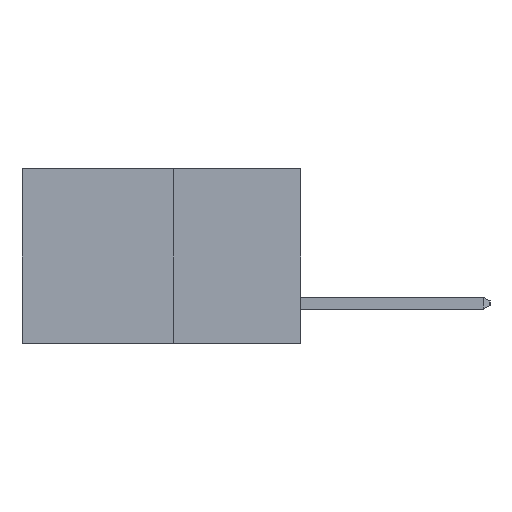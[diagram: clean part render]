
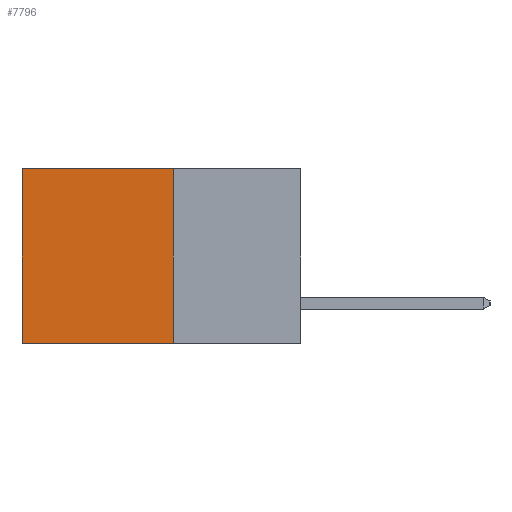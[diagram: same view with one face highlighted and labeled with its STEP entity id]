
A CAD part, left-side view. The second image highlights one B-rep face of the part: STEP entity #7796.
In plain terms, the highlighted planar face has unit normal (-1, 0, 0).
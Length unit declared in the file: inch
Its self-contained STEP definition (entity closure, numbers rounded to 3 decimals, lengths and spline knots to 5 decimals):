
#489 = LINE ( 'NONE', #5922, #3504 ) ;
#704 = LINE ( 'NONE', #11715, #1530 ) ;
#1110 = ORIENTED_EDGE ( 'NONE', *, *, #11844, .F. ) ;
#1530 = VECTOR ( 'NONE', #4206, 39.37008 ) ;
#2030 = FACE_OUTER_BOUND ( 'NONE', #16053, .T. ) ;
#2265 = VECTOR ( 'NONE', #4641, 39.37008 ) ;
#2388 = CARTESIAN_POINT ( 'NONE',  ( 0.277, 0.27, 0. ) ) ;
#2983 = PLANE ( 'NONE',  #4618 ) ;
#3184 = ORIENTED_EDGE ( 'NONE', *, *, #5861, .T. ) ;
#3504 = VECTOR ( 'NONE', #13390, 39.37008 ) ;
#3872 = VERTEX_POINT ( 'NONE', #2388 ) ;
#4088 = CARTESIAN_POINT ( 'NONE',  ( 0.277, 0.59, -0.37 ) ) ;
#4206 = DIRECTION ( 'NONE',  ( 0., 1., 0. ) ) ;
#4225 = DIRECTION ( 'NONE',  ( 0., 0., -1. ) ) ;
#4352 = VERTEX_POINT ( 'NONE', #13667 ) ;
#4618 = AXIS2_PLACEMENT_3D ( 'NONE', #9203, #11729, #4225 ) ;
#4641 = DIRECTION ( 'NONE',  ( 0., 1., 0. ) ) ;
#5349 = DIRECTION ( 'NONE',  ( 0., 0., -1. ) ) ;
#5861 = EDGE_CURVE ( 'NONE', #9383, #13423, #11345, .T. ) ;
#5922 = CARTESIAN_POINT ( 'NONE',  ( 0.277, 0.27, -0.37 ) ) ;
#6138 = CARTESIAN_POINT ( 'NONE',  ( 0.277, 0.59, 0. ) ) ;
#7577 = CARTESIAN_POINT ( 'NONE',  ( 0.277, 0.59, -0.37 ) ) ;
#7591 = VECTOR ( 'NONE', #5349, 39.37008 ) ;
#7796 = ADVANCED_FACE ( 'NONE', ( #2030 ), #2983, .F. ) ;
#9203 = CARTESIAN_POINT ( 'NONE',  ( 0.277, 0.27, -0.37 ) ) ;
#9340 = LINE ( 'NONE', #15729, #2265 ) ;
#9383 = VERTEX_POINT ( 'NONE', #6138 ) ;
#10904 = EDGE_CURVE ( 'NONE', #4352, #13423, #704, .T. ) ;
#11345 = LINE ( 'NONE', #4088, #7591 ) ;
#11715 = CARTESIAN_POINT ( 'NONE',  ( 0.277, 0.27, -0.37 ) ) ;
#11729 = DIRECTION ( 'NONE',  ( 1., 0., 0. ) ) ;
#11844 = EDGE_CURVE ( 'NONE', #3872, #4352, #489, .T. ) ;
#11854 = ORIENTED_EDGE ( 'NONE', *, *, #13147, .T. ) ;
#13147 = EDGE_CURVE ( 'NONE', #3872, #9383, #9340, .T. ) ;
#13390 = DIRECTION ( 'NONE',  ( 0., 0., -1. ) ) ;
#13423 = VERTEX_POINT ( 'NONE', #7577 ) ;
#13538 = ORIENTED_EDGE ( 'NONE', *, *, #10904, .F. ) ;
#13667 = CARTESIAN_POINT ( 'NONE',  ( 0.277, 0.27, -0.37 ) ) ;
#15729 = CARTESIAN_POINT ( 'NONE',  ( 0.277, 0.27, 0. ) ) ;
#16053 = EDGE_LOOP ( 'NONE', ( #3184, #13538, #1110, #11854 ) ) ;
